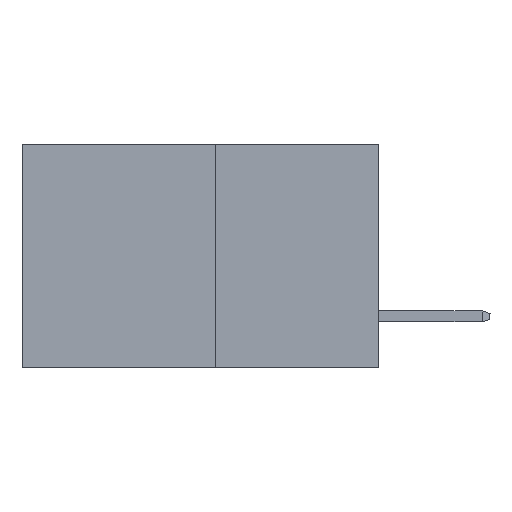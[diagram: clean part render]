
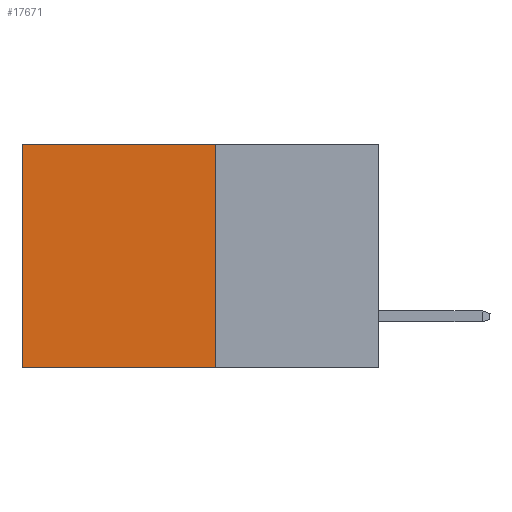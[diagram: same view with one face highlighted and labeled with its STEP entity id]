
A CAD part, left-side view. The second image highlights one B-rep face of the part: STEP entity #17671.
In plain terms, the highlighted planar face has unit normal (-1, 0, 0).
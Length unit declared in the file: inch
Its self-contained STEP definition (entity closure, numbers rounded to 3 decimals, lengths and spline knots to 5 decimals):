
#566 = EDGE_CURVE ( 'NONE', #1186, #18613, #17825, .T. ) ;
#634 = DIRECTION ( 'NONE',  ( 0., 1., 0. ) ) ;
#1186 = VERTEX_POINT ( 'NONE', #28016 ) ;
#1910 = EDGE_CURVE ( 'NONE', #15301, #18613, #10524, .T. ) ;
#1960 = CARTESIAN_POINT ( 'NONE',  ( 0.277, 0.59, 0. ) ) ;
#2038 = CARTESIAN_POINT ( 'NONE',  ( 0.277, 0.27, -0.37 ) ) ;
#2741 = CARTESIAN_POINT ( 'NONE',  ( 0.277, 0.27, 0. ) ) ;
#2787 = DIRECTION ( 'NONE',  ( 1., 0., 0. ) ) ;
#3374 = VECTOR ( 'NONE', #634, 39.37008 ) ;
#4368 = EDGE_CURVE ( 'NONE', #23388, #1186, #8310, .T. ) ;
#4775 = VECTOR ( 'NONE', #27577, 39.37008 ) ;
#5423 = CARTESIAN_POINT ( 'NONE',  ( 0.277, 0.27, -0.37 ) ) ;
#6218 = VECTOR ( 'NONE', #8219, 39.37008 ) ;
#6379 = ORIENTED_EDGE ( 'NONE', *, *, #8183, .T. ) ;
#7951 = CARTESIAN_POINT ( 'NONE',  ( 0.277, 0.59, -0.37 ) ) ;
#8183 = EDGE_CURVE ( 'NONE', #23388, #15301, #15663, .T. ) ;
#8219 = DIRECTION ( 'NONE',  ( 0., 1., 0. ) ) ;
#8310 = LINE ( 'NONE', #5423, #19269 ) ;
#10524 = LINE ( 'NONE', #23242, #4775 ) ;
#11390 = PLANE ( 'NONE',  #16356 ) ;
#13655 = CARTESIAN_POINT ( 'NONE',  ( 0.277, 0.27, -0.37 ) ) ;
#15301 = VERTEX_POINT ( 'NONE', #1960 ) ;
#15663 = LINE ( 'NONE', #2741, #3374 ) ;
#16356 = AXIS2_PLACEMENT_3D ( 'NONE', #13655, #2787, #18042 ) ;
#17634 = ORIENTED_EDGE ( 'NONE', *, *, #566, .F. ) ;
#17671 = ADVANCED_FACE ( 'NONE', ( #18921 ), #11390, .F. ) ;
#17825 = LINE ( 'NONE', #2038, #6218 ) ;
#18042 = DIRECTION ( 'NONE',  ( 0., 0., -1. ) ) ;
#18613 = VERTEX_POINT ( 'NONE', #7951 ) ;
#18921 = FACE_OUTER_BOUND ( 'NONE', #27636, .T. ) ;
#19269 = VECTOR ( 'NONE', #23908, 39.37008 ) ;
#20710 = ORIENTED_EDGE ( 'NONE', *, *, #1910, .T. ) ;
#22398 = ORIENTED_EDGE ( 'NONE', *, *, #4368, .F. ) ;
#23242 = CARTESIAN_POINT ( 'NONE',  ( 0.277, 0.59, -0.37 ) ) ;
#23388 = VERTEX_POINT ( 'NONE', #27995 ) ;
#23908 = DIRECTION ( 'NONE',  ( 0., 0., -1. ) ) ;
#27577 = DIRECTION ( 'NONE',  ( 0., 0., -1. ) ) ;
#27636 = EDGE_LOOP ( 'NONE', ( #20710, #17634, #22398, #6379 ) ) ;
#27995 = CARTESIAN_POINT ( 'NONE',  ( 0.277, 0.27, 0. ) ) ;
#28016 = CARTESIAN_POINT ( 'NONE',  ( 0.277, 0.27, -0.37 ) ) ;
